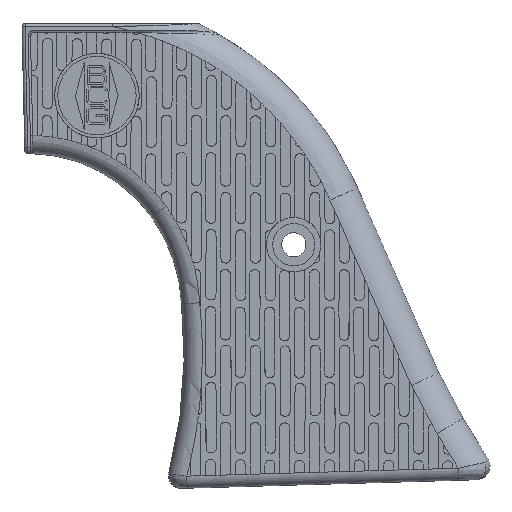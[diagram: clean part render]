
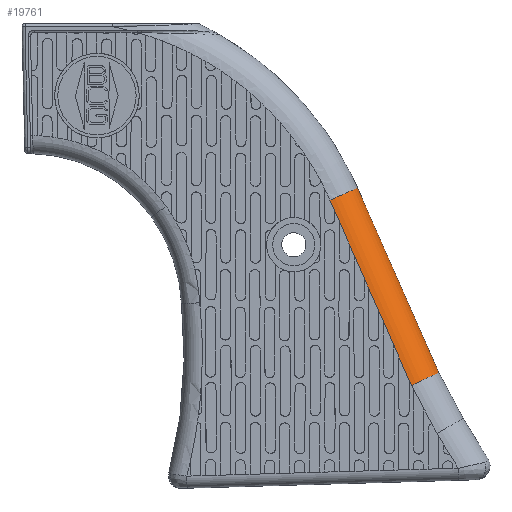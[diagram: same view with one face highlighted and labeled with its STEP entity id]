
A CAD part, left-side view. The second image highlights one B-rep face of the part: STEP entity #19761.
In plain terms, the highlighted cylindrical face has radius 5 mm (diameter 10 mm), a partial arc.
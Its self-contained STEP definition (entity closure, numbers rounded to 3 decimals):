
#27=ELLIPSE('',#20451,5.003,5.);
#125=CYLINDRICAL_SURFACE('',#20450,5.);
#361=CIRCLE('',#20448,5.);
#3199=FACE_OUTER_BOUND('',#4341,.T.);
#4341=EDGE_LOOP('',(#18154,#18155,#18156,#18157,#18158,#18159,#18160,#18161,
#18162,#18163,#18164,#18165,#18166,#18167,#18168));
#4691=LINE('',#25920,#6248);
#4692=LINE('',#25957,#6249);
#4696=LINE('',#25985,#6253);
#4698=LINE('',#26014,#6255);
#4702=LINE('',#26042,#6259);
#4706=LINE('',#26065,#6263);
#5796=LINE('',#36535,#7353);
#5799=LINE('',#36540,#7356);
#5801=LINE('',#36543,#7358);
#5803=LINE('',#36546,#7360);
#5805=LINE('',#36549,#7362);
#5862=LINE('',#36828,#7419);
#5904=LINE('',#37577,#7461);
#6248=VECTOR('',#21072,10.);
#6249=VECTOR('',#21073,10.);
#6253=VECTOR('',#21077,10.);
#6255=VECTOR('',#21079,10.);
#6259=VECTOR('',#21083,10.);
#6263=VECTOR('',#21087,10.);
#7353=VECTOR('',#22629,10.);
#7356=VECTOR('',#22634,10.);
#7358=VECTOR('',#22638,10.);
#7360=VECTOR('',#22642,10.);
#7362=VECTOR('',#22646,10.);
#7419=VECTOR('',#23123,10.);
#7461=VECTOR('',#23337,10.);
#7987=VERTEX_POINT('',#25917);
#7988=VERTEX_POINT('',#25919);
#7995=VERTEX_POINT('',#25951);
#7996=VERTEX_POINT('',#25956);
#8003=VERTEX_POINT('',#25982);
#8004=VERTEX_POINT('',#25984);
#8010=VERTEX_POINT('',#26011);
#8011=VERTEX_POINT('',#26013);
#8018=VERTEX_POINT('',#26039);
#8019=VERTEX_POINT('',#26041);
#8025=VERTEX_POINT('',#26062);
#8026=VERTEX_POINT('',#26064);
#9308=VERTEX_POINT('',#36534);
#9388=VERTEX_POINT('',#37572);
#9389=VERTEX_POINT('',#37576);
#10042=EDGE_CURVE('',#7988,#7987,#4691,.T.);
#10050=EDGE_CURVE('',#7996,#7995,#4692,.T.);
#10058=EDGE_CURVE('',#8004,#8003,#4696,.T.);
#10065=EDGE_CURVE('',#8011,#8010,#4698,.T.);
#10073=EDGE_CURVE('',#8019,#8018,#4702,.T.);
#10080=EDGE_CURVE('',#8026,#8025,#4706,.T.);
#12095=EDGE_CURVE('',#9308,#8026,#5796,.T.);
#12098=EDGE_CURVE('',#8025,#8019,#5799,.T.);
#12100=EDGE_CURVE('',#8018,#8011,#5801,.T.);
#12102=EDGE_CURVE('',#8010,#8004,#5803,.T.);
#12104=EDGE_CURVE('',#8003,#7996,#5805,.T.);
#12221=EDGE_CURVE('',#7995,#7988,#5862,.T.);
#12331=EDGE_CURVE('',#9308,#9388,#361,.T.);
#12333=EDGE_CURVE('',#9389,#9388,#5904,.T.);
#12334=EDGE_CURVE('',#7987,#9389,#27,.T.);
#18154=ORIENTED_EDGE('',*,*,#12333,.T.);
#18155=ORIENTED_EDGE('',*,*,#12331,.F.);
#18156=ORIENTED_EDGE('',*,*,#12095,.T.);
#18157=ORIENTED_EDGE('',*,*,#10080,.T.);
#18158=ORIENTED_EDGE('',*,*,#12098,.T.);
#18159=ORIENTED_EDGE('',*,*,#10073,.T.);
#18160=ORIENTED_EDGE('',*,*,#12100,.T.);
#18161=ORIENTED_EDGE('',*,*,#10065,.T.);
#18162=ORIENTED_EDGE('',*,*,#12102,.T.);
#18163=ORIENTED_EDGE('',*,*,#10058,.T.);
#18164=ORIENTED_EDGE('',*,*,#12104,.T.);
#18165=ORIENTED_EDGE('',*,*,#10050,.T.);
#18166=ORIENTED_EDGE('',*,*,#12221,.T.);
#18167=ORIENTED_EDGE('',*,*,#10042,.T.);
#18168=ORIENTED_EDGE('',*,*,#12334,.T.);
#19761=ADVANCED_FACE('',(#3199),#125,.T.);
#20448=AXIS2_PLACEMENT_3D('',#37573,#23331,#23332);
#20450=AXIS2_PLACEMENT_3D('',#37575,#23335,#23336);
#20451=AXIS2_PLACEMENT_3D('',#37578,#23338,#23339);
#21072=DIRECTION('',(0.,-0.403,-0.915));
#21073=DIRECTION('',(0.,-0.403,-0.915));
#21077=DIRECTION('',(0.,-0.403,-0.915));
#21079=DIRECTION('',(0.,-0.403,-0.915));
#21083=DIRECTION('',(0.,-0.403,-0.915));
#21087=DIRECTION('',(0.,-0.403,-0.915));
#22629=DIRECTION('',(0.,-0.403,-0.915));
#22634=DIRECTION('',(0.,-0.403,-0.915));
#22638=DIRECTION('',(0.,-0.403,-0.915));
#22642=DIRECTION('',(0.,-0.403,-0.915));
#22646=DIRECTION('',(0.,-0.403,-0.915));
#23123=DIRECTION('',(0.,-0.403,-0.915));
#23331=DIRECTION('center_axis',(0.,0.403,
0.915));
#23332=DIRECTION('ref_axis',(-1.,0.,0.));
#23335=DIRECTION('center_axis',(0.,-0.403,
-0.915));
#23336=DIRECTION('ref_axis',(-0.707,-0.647,0.285));
#23337=DIRECTION('',(0.,0.403,0.915));
#23338=DIRECTION('center_axis',(0.,0.437,
0.9));
#23339=DIRECTION('ref_axis',(0.,-0.9,0.437));
#25917=CARTESIAN_POINT('',(-10.692,-53.109,-300.142));
#25919=CARTESIAN_POINT('',(-10.692,-52.715,-299.245));
#25920=CARTESIAN_POINT('',(-10.692,-40.426,-271.334));
#25951=CARTESIAN_POINT('',(-10.692,-51.017,-295.39));
#25956=CARTESIAN_POINT('',(-10.692,-50.137,-293.391));
#25957=CARTESIAN_POINT('',(-10.692,-40.426,-271.334));
#25982=CARTESIAN_POINT('',(-10.692,-48.452,-289.564));
#25984=CARTESIAN_POINT('',(-10.692,-47.697,-287.849));
#25985=CARTESIAN_POINT('',(-10.692,-40.426,-271.334));
#26011=CARTESIAN_POINT('',(-10.692,-45.994,-283.982));
#26013=CARTESIAN_POINT('',(-10.692,-45.304,-282.414));
#26014=CARTESIAN_POINT('',(-10.692,-40.426,-271.334));
#26039=CARTESIAN_POINT('',(-10.692,-43.624,-278.598));
#26041=CARTESIAN_POINT('',(-10.692,-42.848,-276.835));
#26042=CARTESIAN_POINT('',(-10.692,-40.426,-271.334));
#26062=CARTESIAN_POINT('',(-10.692,-41.162,-273.005));
#26064=CARTESIAN_POINT('',(-10.692,-40.413,-271.304));
#26065=CARTESIAN_POINT('',(-10.692,-40.426,-271.334));
#36534=CARTESIAN_POINT('',(-10.692,-39.573,-269.398));
#36535=CARTESIAN_POINT('',(-10.692,-40.426,-271.334));
#36540=CARTESIAN_POINT('',(-10.692,-40.426,-271.334));
#36543=CARTESIAN_POINT('',(-10.692,-40.426,-271.334));
#36546=CARTESIAN_POINT('',(-10.692,-40.426,-271.334));
#36549=CARTESIAN_POINT('',(-10.692,-40.426,-271.334));
#36828=CARTESIAN_POINT('',(-10.692,-40.426,-271.334));
#37572=CARTESIAN_POINT('',(-5.692,-44.15,-267.383));
#37573=CARTESIAN_POINT('Origin',(-5.692,-39.573,-269.398));
#37575=CARTESIAN_POINT('Origin',(-5.692,-40.426,-271.334));
#37576=CARTESIAN_POINT('',(-5.692,-57.611,-297.958));
#37577=CARTESIAN_POINT('',(-5.692,-45.002,-269.319));
#37578=CARTESIAN_POINT('Origin',(-5.692,-53.109,-300.142));
